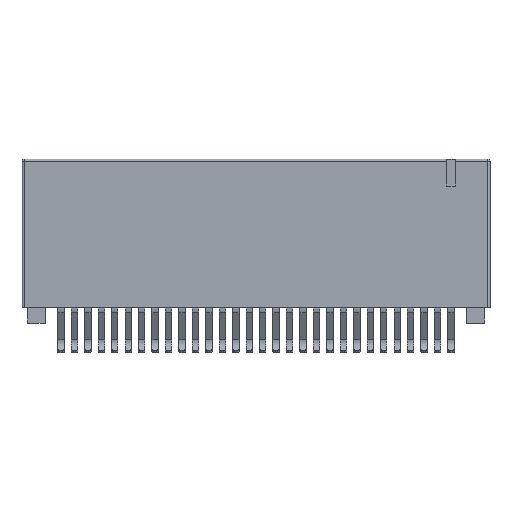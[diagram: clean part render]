
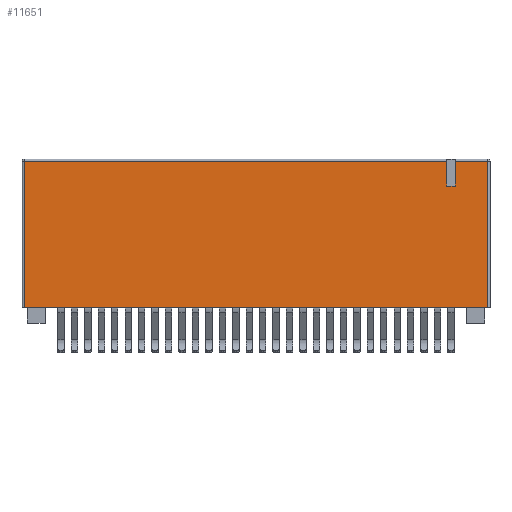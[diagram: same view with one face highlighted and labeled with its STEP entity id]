
A CAD part, top view. The second image highlights one B-rep face of the part: STEP entity #11651.
In plain terms, the highlighted planar face has unit normal (0, 0, 1).
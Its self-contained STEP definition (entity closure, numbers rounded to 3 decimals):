
#86 = CARTESIAN_POINT ( 'NONE',  ( 0.2, 15.3, 0. ) ) ;
#291 = DIRECTION ( 'NONE',  ( 0., 1., 0. ) ) ;
#381 = ORIENTED_EDGE ( 'NONE', *, *, #5682, .F. ) ;
#450 = VERTEX_POINT ( 'NONE', #9656 ) ;
#452 = VERTEX_POINT ( 'NONE', #9420 ) ;
#453 = VERTEX_POINT ( 'NONE', #86 ) ;
#1342 = DIRECTION ( 'NONE',  ( -1., 0., 0. ) ) ;
#1463 = VECTOR ( 'NONE', #7268, 1000. ) ;
#1753 = EDGE_CURVE ( 'NONE', #11239, #16543, #22405, .T. ) ;
#1790 = DIRECTION ( 'NONE',  ( 1., 0., 0. ) ) ;
#2191 = EDGE_CURVE ( 'NONE', #21473, #452, #11121, .T. ) ;
#2915 = CARTESIAN_POINT ( 'NONE',  ( 44., 15.3, 0. ) ) ;
#3285 = CARTESIAN_POINT ( 'NONE',  ( 0.2, 1.5, 0. ) ) ;
#3398 = VECTOR ( 'NONE', #291, 1000. ) ;
#3467 = LINE ( 'NONE', #21860, #1463 ) ;
#3786 = ORIENTED_EDGE ( 'NONE', *, *, #9542, .T. ) ;
#3886 = CARTESIAN_POINT ( 'NONE',  ( 0., 15.5, 0. ) ) ;
#4367 = FACE_OUTER_BOUND ( 'NONE', #5629, .T. ) ;
#4794 = CARTESIAN_POINT ( 'NONE',  ( 0., 15.3, 0. ) ) ;
#5629 = EDGE_LOOP ( 'NONE', ( #10550, #3786, #14068, #18026, #21223, #22367, #6950, #381 ) ) ;
#5682 = EDGE_CURVE ( 'NONE', #452, #16543, #13298, .T. ) ;
#5995 = EDGE_CURVE ( 'NONE', #450, #11239, #3467, .T. ) ;
#6063 = VECTOR ( 'NONE', #21619, 1000. ) ;
#6759 = LINE ( 'NONE', #4794, #17540 ) ;
#6950 = ORIENTED_EDGE ( 'NONE', *, *, #1753, .T. ) ;
#7268 = DIRECTION ( 'NONE',  ( 0., 1., 0. ) ) ;
#8155 = CARTESIAN_POINT ( 'NONE',  ( 0.2, 15.5, 0. ) ) ;
#9420 = CARTESIAN_POINT ( 'NONE',  ( 40.905, 12.95, 0. ) ) ;
#9424 = CARTESIAN_POINT ( 'NONE',  ( 0., 15.3, 0. ) ) ;
#9542 = EDGE_CURVE ( 'NONE', #21473, #21315, #14252, .T. ) ;
#9656 = CARTESIAN_POINT ( 'NONE',  ( 44., 1.5, 0. ) ) ;
#10550 = ORIENTED_EDGE ( 'NONE', *, *, #2191, .F. ) ;
#10646 = VECTOR ( 'NONE', #1790, 1000. ) ;
#10884 = EDGE_CURVE ( 'NONE', #21315, #453, #6759, .T. ) ;
#11121 = LINE ( 'NONE', #18587, #10646 ) ;
#11239 = VERTEX_POINT ( 'NONE', #2915 ) ;
#11345 = CARTESIAN_POINT ( 'NONE',  ( 40.905, 12.95, 0. ) ) ;
#11373 = DIRECTION ( 'NONE',  ( 0., 0., -1. ) ) ;
#11499 = DIRECTION ( 'NONE',  ( -1., 0., 0. ) ) ;
#11651 = ADVANCED_FACE ( 'NONE', ( #4367 ), #11854, .F. ) ;
#11854 = PLANE ( 'NONE',  #21775 ) ;
#12410 = DIRECTION ( 'NONE',  ( 0., 1., 0. ) ) ;
#12881 = VECTOR ( 'NONE', #11499, 1000. ) ;
#13298 = LINE ( 'NONE', #11345, #3398 ) ;
#13566 = DIRECTION ( 'NONE',  ( -1., 0., 0. ) ) ;
#13591 = EDGE_CURVE ( 'NONE', #453, #21218, #15744, .T. ) ;
#14068 = ORIENTED_EDGE ( 'NONE', *, *, #10884, .T. ) ;
#14252 = LINE ( 'NONE', #17932, #20483 ) ;
#15744 = LINE ( 'NONE', #8155, #6063 ) ;
#15855 = EDGE_CURVE ( 'NONE', #450, #21218, #17611, .T. ) ;
#16543 = VERTEX_POINT ( 'NONE', #23942 ) ;
#17540 = VECTOR ( 'NONE', #1342, 1000. ) ;
#17611 = LINE ( 'NONE', #22871, #22206 ) ;
#17932 = CARTESIAN_POINT ( 'NONE',  ( 40.125, 12.95, 0. ) ) ;
#18026 = ORIENTED_EDGE ( 'NONE', *, *, #13591, .T. ) ;
#18587 = CARTESIAN_POINT ( 'NONE',  ( 40.125, 12.95, 0. ) ) ;
#18838 = DIRECTION ( 'NONE',  ( -1., 0., 0. ) ) ;
#20483 = VECTOR ( 'NONE', #12410, 1000. ) ;
#21218 = VERTEX_POINT ( 'NONE', #3285 ) ;
#21223 = ORIENTED_EDGE ( 'NONE', *, *, #15855, .F. ) ;
#21315 = VERTEX_POINT ( 'NONE', #22294 ) ;
#21473 = VERTEX_POINT ( 'NONE', #22769 ) ;
#21619 = DIRECTION ( 'NONE',  ( 0., -1., 0. ) ) ;
#21775 = AXIS2_PLACEMENT_3D ( 'NONE', #3886, #11373, #18838 ) ;
#21860 = CARTESIAN_POINT ( 'NONE',  ( 44., 15.5, 0. ) ) ;
#22206 = VECTOR ( 'NONE', #13566, 1000. ) ;
#22294 = CARTESIAN_POINT ( 'NONE',  ( 40.125, 15.3, 0. ) ) ;
#22367 = ORIENTED_EDGE ( 'NONE', *, *, #5995, .T. ) ;
#22405 = LINE ( 'NONE', #9424, #12881 ) ;
#22769 = CARTESIAN_POINT ( 'NONE',  ( 40.125, 12.95, 0. ) ) ;
#22871 = CARTESIAN_POINT ( 'NONE',  ( 44.2, 1.5, 0. ) ) ;
#23942 = CARTESIAN_POINT ( 'NONE',  ( 40.905, 15.3, 0. ) ) ;
